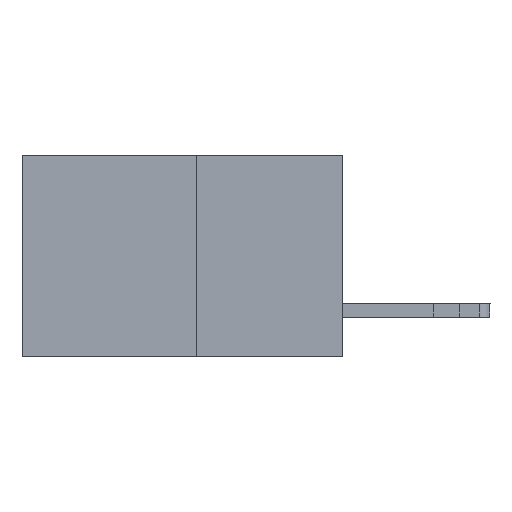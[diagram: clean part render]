
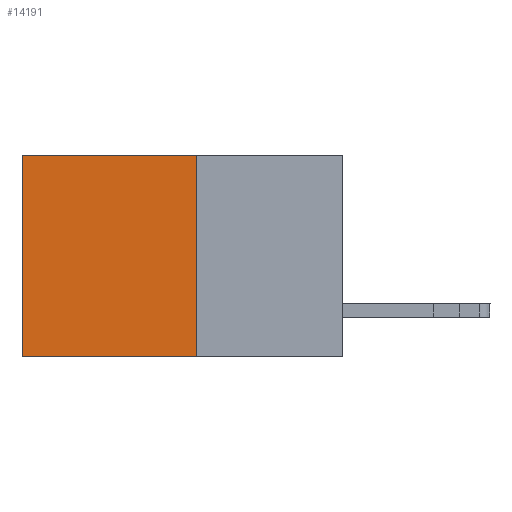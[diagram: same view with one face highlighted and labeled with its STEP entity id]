
A CAD part, left-side view. The second image highlights one B-rep face of the part: STEP entity #14191.
In plain terms, the highlighted planar face has unit normal (-1, 0, 0).
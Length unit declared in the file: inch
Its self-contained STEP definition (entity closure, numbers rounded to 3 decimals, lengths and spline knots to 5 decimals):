
#1342 = VERTEX_POINT ( 'NONE', #22151 ) ;
#1715 = DIRECTION ( 'NONE',  ( 0., 1., 0. ) ) ;
#1892 = VECTOR ( 'NONE', #3007, 39.37008 ) ;
#2371 = CARTESIAN_POINT ( 'NONE',  ( 0.277, 0.27, 0. ) ) ;
#3007 = DIRECTION ( 'NONE',  ( 0., 0., -1. ) ) ;
#3752 = CARTESIAN_POINT ( 'NONE',  ( 0.277, 0.27, -0.37 ) ) ;
#4200 = ORIENTED_EDGE ( 'NONE', *, *, #23306, .T. ) ;
#6464 = DIRECTION ( 'NONE',  ( 0., 1., 0. ) ) ;
#8790 = CARTESIAN_POINT ( 'NONE',  ( 0.277, 0.27, -0.37 ) ) ;
#10022 = CARTESIAN_POINT ( 'NONE',  ( 0.277, 0.59, 0. ) ) ;
#10464 = AXIS2_PLACEMENT_3D ( 'NONE', #3752, #11439, #28886 ) ;
#11439 = DIRECTION ( 'NONE',  ( 1., 0., 0. ) ) ;
#12011 = VERTEX_POINT ( 'NONE', #8790 ) ;
#12066 = ORIENTED_EDGE ( 'NONE', *, *, #22043, .F. ) ;
#12712 = ORIENTED_EDGE ( 'NONE', *, *, #27472, .T. ) ;
#14191 = ADVANCED_FACE ( 'NONE', ( #20955 ), #28787, .F. ) ;
#15636 = CARTESIAN_POINT ( 'NONE',  ( 0.277, 0.59, -0.37 ) ) ;
#16621 = EDGE_CURVE ( 'NONE', #12011, #1342, #16905, .T. ) ;
#16656 = VECTOR ( 'NONE', #1715, 39.37008 ) ;
#16905 = LINE ( 'NONE', #21546, #23560 ) ;
#18151 = VERTEX_POINT ( 'NONE', #2371 ) ;
#19417 = CARTESIAN_POINT ( 'NONE',  ( 0.277, 0.27, 0. ) ) ;
#20955 = FACE_OUTER_BOUND ( 'NONE', #27784, .T. ) ;
#21546 = CARTESIAN_POINT ( 'NONE',  ( 0.277, 0.27, -0.37 ) ) ;
#22040 = LINE ( 'NONE', #15636, #1892 ) ;
#22043 = EDGE_CURVE ( 'NONE', #18151, #12011, #28414, .T. ) ;
#22151 = CARTESIAN_POINT ( 'NONE',  ( 0.277, 0.59, -0.37 ) ) ;
#22959 = ORIENTED_EDGE ( 'NONE', *, *, #16621, .F. ) ;
#23306 = EDGE_CURVE ( 'NONE', #18151, #24112, #23320, .T. ) ;
#23320 = LINE ( 'NONE', #19417, #16656 ) ;
#23560 = VECTOR ( 'NONE', #6464, 39.37008 ) ;
#24112 = VERTEX_POINT ( 'NONE', #10022 ) ;
#24398 = CARTESIAN_POINT ( 'NONE',  ( 0.277, 0.27, -0.37 ) ) ;
#27472 = EDGE_CURVE ( 'NONE', #24112, #1342, #22040, .T. ) ;
#27653 = VECTOR ( 'NONE', #31790, 39.37008 ) ;
#27784 = EDGE_LOOP ( 'NONE', ( #12712, #22959, #12066, #4200 ) ) ;
#28414 = LINE ( 'NONE', #24398, #27653 ) ;
#28787 = PLANE ( 'NONE',  #10464 ) ;
#28886 = DIRECTION ( 'NONE',  ( 0., 0., -1. ) ) ;
#31790 = DIRECTION ( 'NONE',  ( 0., 0., -1. ) ) ;
